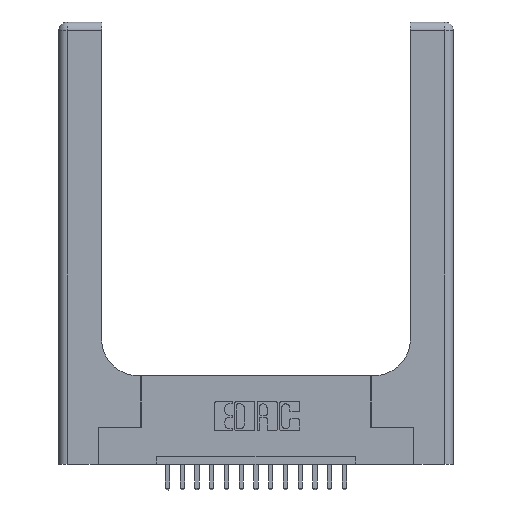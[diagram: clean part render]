
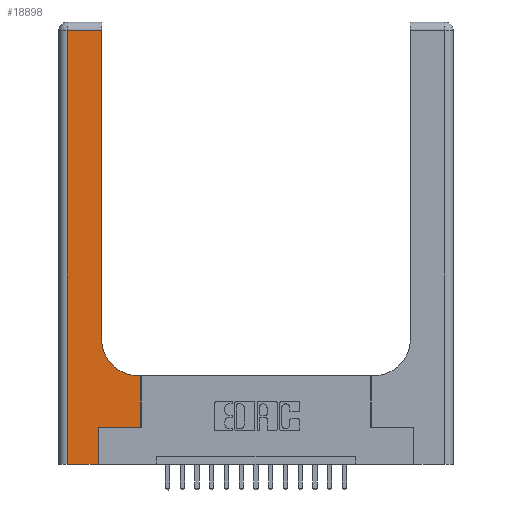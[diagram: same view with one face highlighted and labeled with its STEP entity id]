
A CAD part, top view. The second image highlights one B-rep face of the part: STEP entity #18898.
In plain terms, the highlighted planar face has unit normal (0, 0, 1).
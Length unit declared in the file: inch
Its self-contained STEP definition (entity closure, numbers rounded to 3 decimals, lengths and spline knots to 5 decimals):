
#740 = DIRECTION ( 'NONE',  ( 0., 1., 0. ) ) ;
#761 = AXIS2_PLACEMENT_3D ( 'NONE', #13009, #18998, #4343 ) ;
#1124 = VECTOR ( 'NONE', #16063, 39.37008 ) ;
#1140 = EDGE_CURVE ( 'NONE', #12840, #4470, #9296, .T. ) ;
#1204 = CARTESIAN_POINT ( 'NONE',  ( 0.2915, 0.85, 0.37 ) ) ;
#1217 = VECTOR ( 'NONE', #13603, 39.37008 ) ;
#1295 = EDGE_CURVE ( 'NONE', #4470, #12371, #1536, .T. ) ;
#1450 = CARTESIAN_POINT ( 'NONE',  ( 0.06, 0., 0.37 ) ) ;
#1536 = LINE ( 'NONE', #8470, #12973 ) ;
#1754 = FACE_OUTER_BOUND ( 'NONE', #3385, .T. ) ;
#2135 = CARTESIAN_POINT ( 'NONE',  ( 0.5585, 0.25, 0.37 ) ) ;
#2142 = EDGE_CURVE ( 'NONE', #12371, #18175, #3552, .T. ) ;
#2267 = CARTESIAN_POINT ( 'NONE',  ( 0.269, 0., 0.37 ) ) ;
#2327 = DIRECTION ( 'NONE',  ( 0., 1., 0. ) ) ;
#2484 = CARTESIAN_POINT ( 'NONE',  ( 0., 2.94, 0.37 ) ) ;
#2630 = CARTESIAN_POINT ( 'NONE',  ( 0.2915, 2.94, 0.37 ) ) ;
#3385 = EDGE_LOOP ( 'NONE', ( #3402, #9370, #17411, #15185, #6438, #11381, #15694, #3824, #4502 ) ) ;
#3402 = ORIENTED_EDGE ( 'NONE', *, *, #6222, .T. ) ;
#3552 = LINE ( 'NONE', #7480, #18684 ) ;
#3824 = ORIENTED_EDGE ( 'NONE', *, *, #11942, .T. ) ;
#4343 = DIRECTION ( 'NONE',  ( -1., 0., 0. ) ) ;
#4470 = VERTEX_POINT ( 'NONE', #14500 ) ;
#4502 = ORIENTED_EDGE ( 'NONE', *, *, #14416, .T. ) ;
#4711 = LINE ( 'NONE', #9107, #13199 ) ;
#5842 = VERTEX_POINT ( 'NONE', #1204 ) ;
#6007 = EDGE_CURVE ( 'NONE', #17655, #14238, #17600, .T. ) ;
#6222 = EDGE_CURVE ( 'NONE', #5842, #12840, #6835, .T. ) ;
#6438 = ORIENTED_EDGE ( 'NONE', *, *, #16804, .T. ) ;
#6698 = DIRECTION ( 'NONE',  ( -1., 0., 0. ) ) ;
#6835 = LINE ( 'NONE', #12617, #12311 ) ;
#6902 = CIRCLE ( 'NONE', #17592, 0.25 ) ;
#7439 = VERTEX_POINT ( 'NONE', #14080 ) ;
#7480 = CARTESIAN_POINT ( 'NONE',  ( 0., 0., 0.37 ) ) ;
#7581 = DIRECTION ( 'NONE',  ( -1., 0., 0. ) ) ;
#8470 = CARTESIAN_POINT ( 'NONE',  ( 0.06, 3., 0.37 ) ) ;
#8529 = EDGE_CURVE ( 'NONE', #14238, #16963, #15194, .T. ) ;
#8535 = DIRECTION ( 'NONE',  ( 0., -1., 0. ) ) ;
#8842 = DIRECTION ( 'NONE',  ( 1., 0., 0. ) ) ;
#9107 = CARTESIAN_POINT ( 'NONE',  ( 0.2915, 0.6, 0.37 ) ) ;
#9117 = CARTESIAN_POINT ( 'NONE',  ( 0.269, 0.25, 0.37 ) ) ;
#9296 = LINE ( 'NONE', #2484, #10677 ) ;
#9370 = ORIENTED_EDGE ( 'NONE', *, *, #1140, .T. ) ;
#9562 = LINE ( 'NONE', #2267, #10931 ) ;
#10677 = VECTOR ( 'NONE', #6698, 39.37008 ) ;
#10745 = DIRECTION ( 'NONE',  ( 0., 0., -1. ) ) ;
#10931 = VECTOR ( 'NONE', #740, 39.37008 ) ;
#11381 = ORIENTED_EDGE ( 'NONE', *, *, #6007, .T. ) ;
#11628 = PLANE ( 'NONE',  #761 ) ;
#11640 = CARTESIAN_POINT ( 'NONE',  ( 0.5585, 0.25, 0.37 ) ) ;
#11942 = EDGE_CURVE ( 'NONE', #16963, #7439, #4711, .T. ) ;
#12311 = VECTOR ( 'NONE', #2327, 39.37008 ) ;
#12371 = VERTEX_POINT ( 'NONE', #1450 ) ;
#12617 = CARTESIAN_POINT ( 'NONE',  ( 0.2915, 3., 0.37 ) ) ;
#12840 = VERTEX_POINT ( 'NONE', #2630 ) ;
#12973 = VECTOR ( 'NONE', #8535, 39.37008 ) ;
#13009 = CARTESIAN_POINT ( 'NONE',  ( 0., 3., 0.37 ) ) ;
#13032 = CARTESIAN_POINT ( 'NONE',  ( 0.269, 0., 0.37 ) ) ;
#13199 = VECTOR ( 'NONE', #7581, 39.37008 ) ;
#13279 = CARTESIAN_POINT ( 'NONE',  ( 0.269, 0.25, 0.37 ) ) ;
#13603 = DIRECTION ( 'NONE',  ( 0., 1., 0. ) ) ;
#13735 = CARTESIAN_POINT ( 'NONE',  ( 0.5415, 0.85, 0.37 ) ) ;
#14080 = CARTESIAN_POINT ( 'NONE',  ( 0.5415, 0.6, 0.37 ) ) ;
#14238 = VERTEX_POINT ( 'NONE', #11640 ) ;
#14416 = EDGE_CURVE ( 'NONE', #7439, #5842, #6902, .T. ) ;
#14500 = CARTESIAN_POINT ( 'NONE',  ( 0.06, 2.94, 0.37 ) ) ;
#15185 = ORIENTED_EDGE ( 'NONE', *, *, #2142, .T. ) ;
#15194 = LINE ( 'NONE', #2135, #1217 ) ;
#15694 = ORIENTED_EDGE ( 'NONE', *, *, #8529, .T. ) ;
#15983 = CARTESIAN_POINT ( 'NONE',  ( 0.5585, 0.6, 0.37 ) ) ;
#16063 = DIRECTION ( 'NONE',  ( 1., 0., 0. ) ) ;
#16804 = EDGE_CURVE ( 'NONE', #18175, #17655, #9562, .T. ) ;
#16820 = DIRECTION ( 'NONE',  ( 1., 0., 0. ) ) ;
#16963 = VERTEX_POINT ( 'NONE', #15983 ) ;
#17411 = ORIENTED_EDGE ( 'NONE', *, *, #1295, .T. ) ;
#17592 = AXIS2_PLACEMENT_3D ( 'NONE', #13735, #10745, #16820 ) ;
#17600 = LINE ( 'NONE', #13279, #1124 ) ;
#17655 = VERTEX_POINT ( 'NONE', #9117 ) ;
#18175 = VERTEX_POINT ( 'NONE', #13032 ) ;
#18684 = VECTOR ( 'NONE', #8842, 39.37008 ) ;
#18898 = ADVANCED_FACE ( 'NONE', ( #1754 ), #11628, .F. ) ;
#18998 = DIRECTION ( 'NONE',  ( 0., 0., -1. ) ) ;
